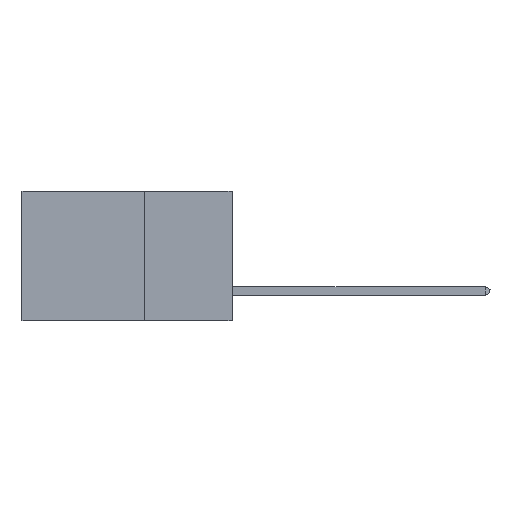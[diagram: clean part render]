
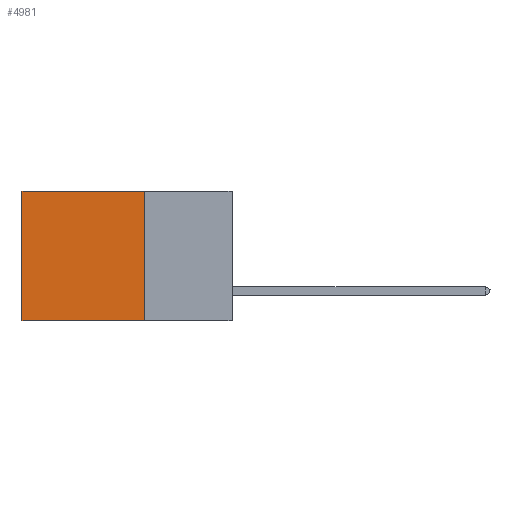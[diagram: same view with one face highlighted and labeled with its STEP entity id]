
A CAD part, left-side view. The second image highlights one B-rep face of the part: STEP entity #4981.
In plain terms, the highlighted planar face has unit normal (-1, 0, 0).
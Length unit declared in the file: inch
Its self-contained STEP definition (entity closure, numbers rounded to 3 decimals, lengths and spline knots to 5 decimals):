
#1151 = EDGE_LOOP ( 'NONE', ( #5792, #8805, #5480, #5748 ) ) ;
#1228 = CARTESIAN_POINT ( 'NONE',  ( 0.2875, 0.6, 0. ) ) ;
#1546 = CARTESIAN_POINT ( 'NONE',  ( 0.2875, 0.25, -0.37 ) ) ;
#1796 = CARTESIAN_POINT ( 'NONE',  ( 0.2875, 0.25, 0. ) ) ;
#3269 = DIRECTION ( 'NONE',  ( 0., 1., 0. ) ) ;
#3343 = DIRECTION ( 'NONE',  ( 0., 0., -1. ) ) ;
#3451 = CARTESIAN_POINT ( 'NONE',  ( 0.2875, 0.6, -0.37 ) ) ;
#3770 = DIRECTION ( 'NONE',  ( 0., 0., -1. ) ) ;
#4053 = VECTOR ( 'NONE', #5547, 39.37008 ) ;
#4315 = CARTESIAN_POINT ( 'NONE',  ( 0.2875, 0.25, 0. ) ) ;
#4981 = ADVANCED_FACE ( 'NONE', ( #10196 ), #11676, .F. ) ;
#5480 = ORIENTED_EDGE ( 'NONE', *, *, #19520, .F. ) ;
#5547 = DIRECTION ( 'NONE',  ( 0., 1., 0. ) ) ;
#5748 = ORIENTED_EDGE ( 'NONE', *, *, #9064, .T. ) ;
#5792 = ORIENTED_EDGE ( 'NONE', *, *, #12553, .T. ) ;
#6005 = VERTEX_POINT ( 'NONE', #3451 ) ;
#7545 = EDGE_CURVE ( 'NONE', #16789, #6005, #9608, .T. ) ;
#7938 = VECTOR ( 'NONE', #3343, 39.37008 ) ;
#8805 = ORIENTED_EDGE ( 'NONE', *, *, #7545, .F. ) ;
#9064 = EDGE_CURVE ( 'NONE', #10915, #14378, #20189, .T. ) ;
#9342 = VECTOR ( 'NONE', #3269, 39.37008 ) ;
#9608 = LINE ( 'NONE', #10279, #9342 ) ;
#9900 = DIRECTION ( 'NONE',  ( 1., 0., 0. ) ) ;
#9955 = VECTOR ( 'NONE', #19670, 39.37008 ) ;
#10196 = FACE_OUTER_BOUND ( 'NONE', #1151, .T. ) ;
#10279 = CARTESIAN_POINT ( 'NONE',  ( 0.2875, 0.25, -0.37 ) ) ;
#10915 = VERTEX_POINT ( 'NONE', #4315 ) ;
#11676 = PLANE ( 'NONE',  #19732 ) ;
#11730 = LINE ( 'NONE', #18367, #9955 ) ;
#12553 = EDGE_CURVE ( 'NONE', #14378, #6005, #18065, .T. ) ;
#14378 = VERTEX_POINT ( 'NONE', #1228 ) ;
#14465 = CARTESIAN_POINT ( 'NONE',  ( 0.2875, 0.6, 0. ) ) ;
#16099 = CARTESIAN_POINT ( 'NONE',  ( 0.2875, 0.25, 0. ) ) ;
#16789 = VERTEX_POINT ( 'NONE', #1546 ) ;
#18065 = LINE ( 'NONE', #14465, #7938 ) ;
#18367 = CARTESIAN_POINT ( 'NONE',  ( 0.2875, 0.25, 0. ) ) ;
#19520 = EDGE_CURVE ( 'NONE', #10915, #16789, #11730, .T. ) ;
#19670 = DIRECTION ( 'NONE',  ( 0., 0., -1. ) ) ;
#19732 = AXIS2_PLACEMENT_3D ( 'NONE', #1796, #9900, #3770 ) ;
#20189 = LINE ( 'NONE', #16099, #4053 ) ;
